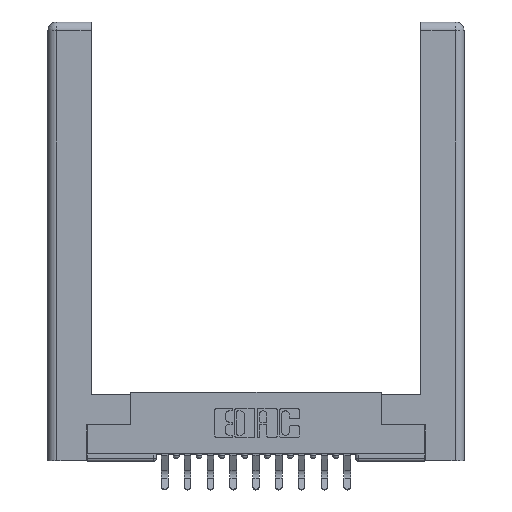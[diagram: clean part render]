
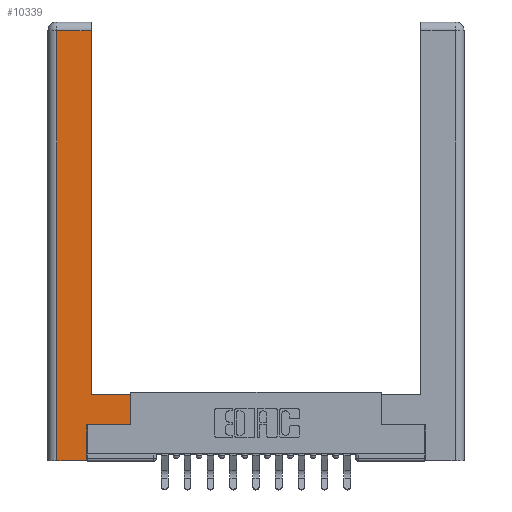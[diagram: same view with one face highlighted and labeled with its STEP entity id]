
A CAD part, top view. The second image highlights one B-rep face of the part: STEP entity #10339.
In plain terms, the highlighted planar face has unit normal (0, 0, 1).
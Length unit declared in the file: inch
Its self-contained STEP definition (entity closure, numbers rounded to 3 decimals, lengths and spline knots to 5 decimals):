
#45 = CARTESIAN_POINT ( 'NONE',  ( 0.565, 0.45, 0. ) ) ;
#180 = VECTOR ( 'NONE', #3556, 39.37008 ) ;
#279 = CARTESIAN_POINT ( 'NONE',  ( 0.265, 0., 0. ) ) ;
#321 = ORIENTED_EDGE ( 'NONE', *, *, #6280, .T. ) ;
#408 = DIRECTION ( 'NONE',  ( 1., 0., 0. ) ) ;
#437 = VECTOR ( 'NONE', #5391, 39.37008 ) ;
#450 = ORIENTED_EDGE ( 'NONE', *, *, #14279, .T. ) ;
#470 = VERTEX_POINT ( 'NONE', #5974 ) ;
#569 = DIRECTION ( 'NONE',  ( -1., 0., 0. ) ) ;
#836 = EDGE_CURVE ( 'NONE', #10997, #14595, #7769, .T. ) ;
#898 = EDGE_CURVE ( 'NONE', #8173, #953, #5420, .T. ) ;
#912 = ORIENTED_EDGE ( 'NONE', *, *, #898, .T. ) ;
#953 = VERTEX_POINT ( 'NONE', #3652 ) ;
#1232 = LINE ( 'NONE', #45, #180 ) ;
#2202 = DIRECTION ( 'NONE',  ( -1., 0., 0. ) ) ;
#2342 = EDGE_CURVE ( 'NONE', #12361, #470, #10101, .T. ) ;
#2602 = VECTOR ( 'NONE', #569, 39.37008 ) ;
#2770 = VECTOR ( 'NONE', #6635, 39.37008 ) ;
#3087 = CARTESIAN_POINT ( 'NONE',  ( 0.0615, 2.94, 0. ) ) ;
#3556 = DIRECTION ( 'NONE',  ( 0., 1., 0. ) ) ;
#3652 = CARTESIAN_POINT ( 'NONE',  ( 0.295, 2.94, 0. ) ) ;
#3660 = LINE ( 'NONE', #6203, #2602 ) ;
#4055 = CARTESIAN_POINT ( 'NONE',  ( 0.565, 0.245, 0. ) ) ;
#4203 = AXIS2_PLACEMENT_3D ( 'NONE', #5690, #10075, #2202 ) ;
#4423 = DIRECTION ( 'NONE',  ( 0., 1., 0. ) ) ;
#4471 = DIRECTION ( 'NONE',  ( 1., 0., 0. ) ) ;
#4635 = VERTEX_POINT ( 'NONE', #5788 ) ;
#4942 = LINE ( 'NONE', #11108, #13732 ) ;
#5123 = ORIENTED_EDGE ( 'NONE', *, *, #12830, .T. ) ;
#5337 = EDGE_CURVE ( 'NONE', #470, #4635, #1232, .T. ) ;
#5391 = DIRECTION ( 'NONE',  ( 0., 1., 0. ) ) ;
#5420 = LINE ( 'NONE', #7885, #9547 ) ;
#5690 = CARTESIAN_POINT ( 'NONE',  ( 0., 0., 0. ) ) ;
#5703 = ORIENTED_EDGE ( 'NONE', *, *, #13636, .T. ) ;
#5777 = VECTOR ( 'NONE', #4471, 39.37008 ) ;
#5788 = CARTESIAN_POINT ( 'NONE',  ( 0.565, 0.45, 0. ) ) ;
#5815 = LINE ( 'NONE', #3087, #2770 ) ;
#5974 = CARTESIAN_POINT ( 'NONE',  ( 0.565, 0.245, 0. ) ) ;
#6137 = CARTESIAN_POINT ( 'NONE',  ( 0.0615, 2.94, 0. ) ) ;
#6203 = CARTESIAN_POINT ( 'NONE',  ( 0.295, 0.45, 0. ) ) ;
#6280 = EDGE_CURVE ( 'NONE', #8386, #10997, #4942, .T. ) ;
#6635 = DIRECTION ( 'NONE',  ( -1., 0., 0. ) ) ;
#6810 = EDGE_LOOP ( 'NONE', ( #912, #450, #321, #10661, #5703, #14720, #9340, #5123 ) ) ;
#6856 = CARTESIAN_POINT ( 'NONE',  ( 0.265, 0.245, 0. ) ) ;
#7769 = LINE ( 'NONE', #13733, #5777 ) ;
#7885 = CARTESIAN_POINT ( 'NONE',  ( 0.295, 3., 0. ) ) ;
#8173 = VERTEX_POINT ( 'NONE', #10369 ) ;
#8386 = VERTEX_POINT ( 'NONE', #6137 ) ;
#8901 = CARTESIAN_POINT ( 'NONE',  ( 0.265, 0.245, 0. ) ) ;
#9340 = ORIENTED_EDGE ( 'NONE', *, *, #5337, .T. ) ;
#9547 = VECTOR ( 'NONE', #4423, 39.37008 ) ;
#10075 = DIRECTION ( 'NONE',  ( 0., 0., -1. ) ) ;
#10101 = LINE ( 'NONE', #4055, #12614 ) ;
#10339 = ADVANCED_FACE ( 'NONE', ( #11283 ), #11410, .F. ) ;
#10369 = CARTESIAN_POINT ( 'NONE',  ( 0.295, 0.45, 0. ) ) ;
#10661 = ORIENTED_EDGE ( 'NONE', *, *, #836, .T. ) ;
#10997 = VERTEX_POINT ( 'NONE', #11439 ) ;
#11108 = CARTESIAN_POINT ( 'NONE',  ( 0.0615, 0., 0. ) ) ;
#11283 = FACE_OUTER_BOUND ( 'NONE', #6810, .T. ) ;
#11410 = PLANE ( 'NONE',  #4203 ) ;
#11439 = CARTESIAN_POINT ( 'NONE',  ( 0.0615, 0., 0. ) ) ;
#11547 = LINE ( 'NONE', #8901, #437 ) ;
#12361 = VERTEX_POINT ( 'NONE', #6856 ) ;
#12614 = VECTOR ( 'NONE', #408, 39.37008 ) ;
#12830 = EDGE_CURVE ( 'NONE', #4635, #8173, #3660, .T. ) ;
#13636 = EDGE_CURVE ( 'NONE', #14595, #12361, #11547, .T. ) ;
#13732 = VECTOR ( 'NONE', #14623, 39.37008 ) ;
#13733 = CARTESIAN_POINT ( 'NONE',  ( 0.265, 0., 0. ) ) ;
#14279 = EDGE_CURVE ( 'NONE', #953, #8386, #5815, .T. ) ;
#14595 = VERTEX_POINT ( 'NONE', #279 ) ;
#14623 = DIRECTION ( 'NONE',  ( 0., -1., 0. ) ) ;
#14720 = ORIENTED_EDGE ( 'NONE', *, *, #2342, .T. ) ;
